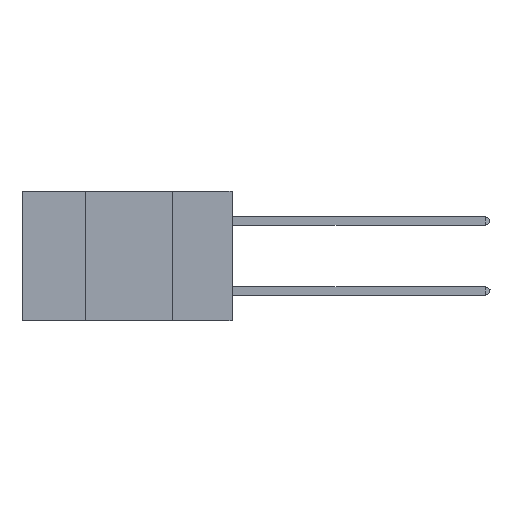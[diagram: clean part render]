
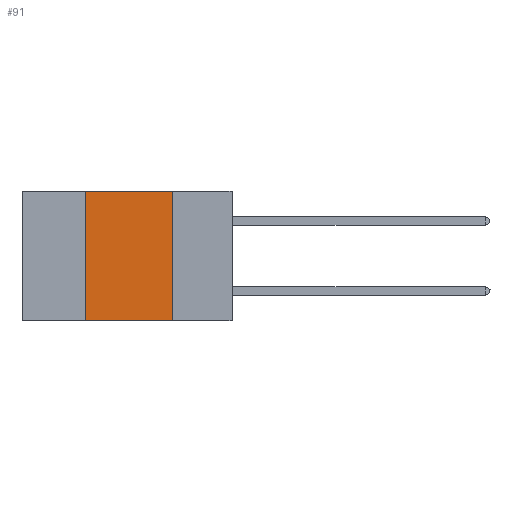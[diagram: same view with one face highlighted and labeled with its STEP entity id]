
A CAD part, left-side view. The second image highlights one B-rep face of the part: STEP entity #91.
In plain terms, the highlighted planar face has unit normal (-1, 0, 0).
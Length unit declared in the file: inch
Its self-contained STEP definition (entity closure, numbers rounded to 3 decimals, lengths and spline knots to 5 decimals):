
#91 = ADVANCED_FACE ( 'NONE', ( #8543 ), #14604, .F. ) ;
#145 = VERTEX_POINT ( 'NONE', #7447 ) ;
#621 = ORIENTED_EDGE ( 'NONE', *, *, #17202, .F. ) ;
#1052 = ORIENTED_EDGE ( 'NONE', *, *, #17281, .F. ) ;
#1107 = DIRECTION ( 'NONE',  ( 0., 0., -1. ) ) ;
#1145 = ORIENTED_EDGE ( 'NONE', *, *, #10045, .T. ) ;
#1220 = ORIENTED_EDGE ( 'NONE', *, *, #16656, .F. ) ;
#1817 = VECTOR ( 'NONE', #13014, 39.37008 ) ;
#2253 = CARTESIAN_POINT ( 'NONE',  ( 0., 0.6, -0.37 ) ) ;
#2275 = DIRECTION ( 'NONE',  ( 1., 0., 0. ) ) ;
#3144 = LINE ( 'NONE', #13218, #6762 ) ;
#4026 = VECTOR ( 'NONE', #14762, 39.37008 ) ;
#4662 = LINE ( 'NONE', #13454, #4026 ) ;
#6286 = CARTESIAN_POINT ( 'NONE',  ( 0., 0.6, 0. ) ) ;
#6762 = VECTOR ( 'NONE', #1107, 39.37008 ) ;
#7401 = VERTEX_POINT ( 'NONE', #16206 ) ;
#7447 = CARTESIAN_POINT ( 'NONE',  ( 0., 0.17, 0. ) ) ;
#8543 = FACE_OUTER_BOUND ( 'NONE', #15036, .T. ) ;
#8638 = LINE ( 'NONE', #17243, #12166 ) ;
#8788 = AXIS2_PLACEMENT_3D ( 'NONE', #6286, #2275, #12952 ) ;
#10045 = EDGE_CURVE ( 'NONE', #13993, #13747, #16005, .T. ) ;
#10746 = DIRECTION ( 'NONE',  ( 0., -1., 0. ) ) ;
#12166 = VECTOR ( 'NONE', #10746, 39.37008 ) ;
#12952 = DIRECTION ( 'NONE',  ( 0., 0., -1. ) ) ;
#13014 = DIRECTION ( 'NONE',  ( 0., -1., 0. ) ) ;
#13218 = CARTESIAN_POINT ( 'NONE',  ( 0., 0.17, 0. ) ) ;
#13454 = CARTESIAN_POINT ( 'NONE',  ( 0., 0.42, 0. ) ) ;
#13747 = VERTEX_POINT ( 'NONE', #15349 ) ;
#13993 = VERTEX_POINT ( 'NONE', #17105 ) ;
#14604 = PLANE ( 'NONE',  #8788 ) ;
#14762 = DIRECTION ( 'NONE',  ( 0., 0., 1. ) ) ;
#15036 = EDGE_LOOP ( 'NONE', ( #621, #1052, #1220, #1145 ) ) ;
#15349 = CARTESIAN_POINT ( 'NONE',  ( 0., 0.17, -0.37 ) ) ;
#16005 = LINE ( 'NONE', #2253, #1817 ) ;
#16206 = CARTESIAN_POINT ( 'NONE',  ( 0., 0.42, 0. ) ) ;
#16656 = EDGE_CURVE ( 'NONE', #13993, #7401, #4662, .T. ) ;
#17105 = CARTESIAN_POINT ( 'NONE',  ( 0., 0.42, -0.37 ) ) ;
#17202 = EDGE_CURVE ( 'NONE', #145, #13747, #3144, .T. ) ;
#17243 = CARTESIAN_POINT ( 'NONE',  ( 0., 0.6, 0. ) ) ;
#17281 = EDGE_CURVE ( 'NONE', #7401, #145, #8638, .T. ) ;
